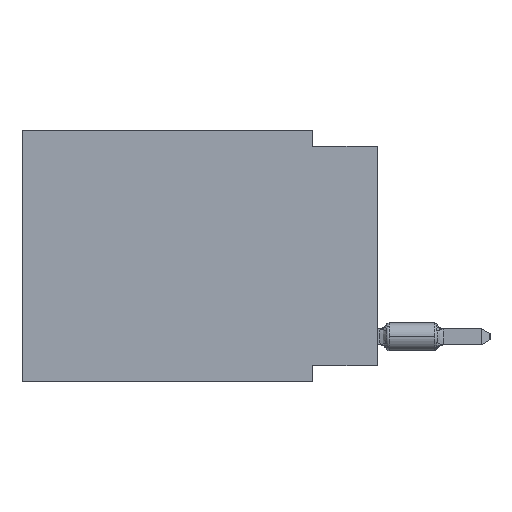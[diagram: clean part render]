
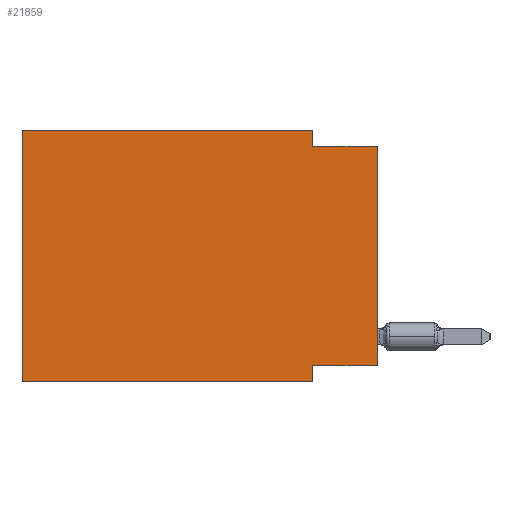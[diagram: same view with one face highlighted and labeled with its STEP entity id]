
A CAD part, left-side view. The second image highlights one B-rep face of the part: STEP entity #21859.
In plain terms, the highlighted planar face has unit normal (-1, 0, 0).
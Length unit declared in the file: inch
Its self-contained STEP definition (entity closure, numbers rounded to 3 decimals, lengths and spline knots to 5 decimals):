
#208 = VECTOR ( 'NONE', #44179, 39.37008 ) ;
#1492 = LINE ( 'NONE', #52611, #20256 ) ;
#1906 = AXIS2_PLACEMENT_3D ( 'NONE', #7426, #24451, #46232 ) ;
#2464 = CARTESIAN_POINT ( 'NONE',  ( 0., 0.1, 0. ) ) ;
#2837 = LINE ( 'NONE', #27424, #37373 ) ;
#4570 = VERTEX_POINT ( 'NONE', #40734 ) ;
#6290 = CARTESIAN_POINT ( 'NONE',  ( 0., 0.55, -0.39 ) ) ;
#7319 = VERTEX_POINT ( 'NONE', #31480 ) ;
#7426 = CARTESIAN_POINT ( 'NONE',  ( 0., 0.55, 0. ) ) ;
#7896 = VECTOR ( 'NONE', #26148, 39.37008 ) ;
#9768 = EDGE_CURVE ( 'NONE', #31215, #24307, #43142, .T. ) ;
#10838 = LINE ( 'NONE', #2464, #33099 ) ;
#11438 = ORIENTED_EDGE ( 'NONE', *, *, #19159, .F. ) ;
#12183 = DIRECTION ( 'NONE',  ( 0., 0., -1. ) ) ;
#13481 = ORIENTED_EDGE ( 'NONE', *, *, #9768, .F. ) ;
#13625 = ORIENTED_EDGE ( 'NONE', *, *, #42346, .F. ) ;
#14587 = DIRECTION ( 'NONE',  ( 0., 0., 1. ) ) ;
#16896 = PLANE ( 'NONE',  #1906 ) ;
#17817 = VERTEX_POINT ( 'NONE', #29247 ) ;
#18463 = CARTESIAN_POINT ( 'NONE',  ( 0., 0.55, -0.39 ) ) ;
#18502 = CARTESIAN_POINT ( 'NONE',  ( 0., 0., -0.025 ) ) ;
#19159 = EDGE_CURVE ( 'NONE', #7319, #49492, #33444, .T. ) ;
#20256 = VECTOR ( 'NONE', #31398, 39.37008 ) ;
#21763 = VERTEX_POINT ( 'NONE', #6290 ) ;
#21859 = ADVANCED_FACE ( 'NONE', ( #32302 ), #16896, .F. ) ;
#22657 = VECTOR ( 'NONE', #34756, 39.37008 ) ;
#23011 = LINE ( 'NONE', #34791, #7896 ) ;
#24307 = VERTEX_POINT ( 'NONE', #27100 ) ;
#24451 = DIRECTION ( 'NONE',  ( 1., 0., 0. ) ) ;
#24679 = ORIENTED_EDGE ( 'NONE', *, *, #53089, .F. ) ;
#24934 = ORIENTED_EDGE ( 'NONE', *, *, #29806, .F. ) ;
#26148 = DIRECTION ( 'NONE',  ( 0., 0., 1. ) ) ;
#27100 = CARTESIAN_POINT ( 'NONE',  ( 0., 0., -0.025 ) ) ;
#27424 = CARTESIAN_POINT ( 'NONE',  ( 0., 0., 0. ) ) ;
#29066 = ORIENTED_EDGE ( 'NONE', *, *, #44127, .F. ) ;
#29247 = CARTESIAN_POINT ( 'NONE',  ( 0., 0., -0.365 ) ) ;
#29806 = EDGE_CURVE ( 'NONE', #17817, #7319, #1492, .T. ) ;
#31215 = VERTEX_POINT ( 'NONE', #54087 ) ;
#31257 = DIRECTION ( 'NONE',  ( 0., 0., -1. ) ) ;
#31398 = DIRECTION ( 'NONE',  ( 0., 1., 0. ) ) ;
#31480 = CARTESIAN_POINT ( 'NONE',  ( 0., 0.1, -0.365 ) ) ;
#32230 = VECTOR ( 'NONE', #12183, 39.37008 ) ;
#32302 = FACE_OUTER_BOUND ( 'NONE', #35509, .T. ) ;
#33099 = VECTOR ( 'NONE', #31257, 39.37008 ) ;
#33444 = LINE ( 'NONE', #50474, #32230 ) ;
#34756 = DIRECTION ( 'NONE',  ( 0., -1., 0. ) ) ;
#34791 = CARTESIAN_POINT ( 'NONE',  ( 0., 0.55, 0. ) ) ;
#35509 = EDGE_LOOP ( 'NONE', ( #53178, #13481, #24679, #29066, #13625, #39633, #11438, #24934 ) ) ;
#36051 = CARTESIAN_POINT ( 'NONE',  ( 0., 0.1, 0. ) ) ;
#36852 = VERTEX_POINT ( 'NONE', #36051 ) ;
#37041 = DIRECTION ( 'NONE',  ( 0., -1., 0. ) ) ;
#37373 = VECTOR ( 'NONE', #14587, 39.37008 ) ;
#39633 = ORIENTED_EDGE ( 'NONE', *, *, #52634, .T. ) ;
#40734 = CARTESIAN_POINT ( 'NONE',  ( 0., 0.55, 0. ) ) ;
#42346 = EDGE_CURVE ( 'NONE', #21763, #4570, #23011, .T. ) ;
#42814 = EDGE_CURVE ( 'NONE', #17817, #24307, #2837, .T. ) ;
#43142 = LINE ( 'NONE', #18502, #22657 ) ;
#43909 = LINE ( 'NONE', #18463, #208 ) ;
#44127 = EDGE_CURVE ( 'NONE', #4570, #36852, #49041, .T. ) ;
#44179 = DIRECTION ( 'NONE',  ( 0., -1., 0. ) ) ;
#44870 = CARTESIAN_POINT ( 'NONE',  ( 0., 0.55, 0. ) ) ;
#45454 = VECTOR ( 'NONE', #37041, 39.37008 ) ;
#46232 = DIRECTION ( 'NONE',  ( 0., 0., -1. ) ) ;
#49041 = LINE ( 'NONE', #44870, #45454 ) ;
#49492 = VERTEX_POINT ( 'NONE', #55072 ) ;
#50474 = CARTESIAN_POINT ( 'NONE',  ( 0., 0.1, -0.39 ) ) ;
#52611 = CARTESIAN_POINT ( 'NONE',  ( 0., 0., -0.365 ) ) ;
#52634 = EDGE_CURVE ( 'NONE', #21763, #49492, #43909, .T. ) ;
#53089 = EDGE_CURVE ( 'NONE', #36852, #31215, #10838, .T. ) ;
#53178 = ORIENTED_EDGE ( 'NONE', *, *, #42814, .T. ) ;
#54087 = CARTESIAN_POINT ( 'NONE',  ( 0., 0.1, -0.025 ) ) ;
#55072 = CARTESIAN_POINT ( 'NONE',  ( 0., 0.1, -0.39 ) ) ;
